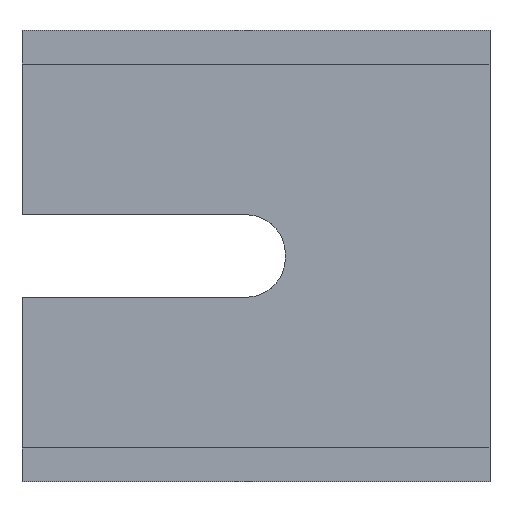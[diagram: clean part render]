
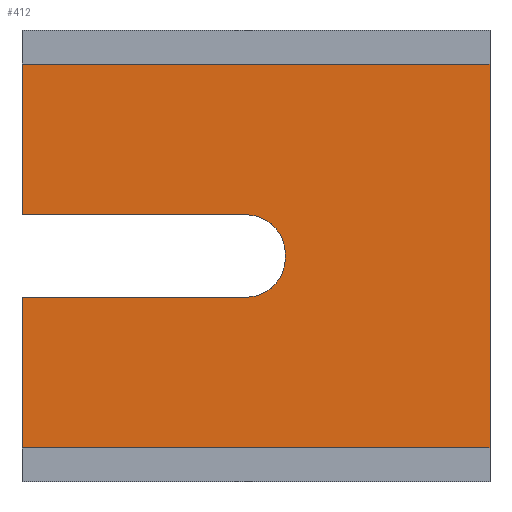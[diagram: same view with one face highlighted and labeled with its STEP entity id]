
A CAD part, front view. The second image highlights one B-rep face of the part: STEP entity #412.
In plain terms, the highlighted planar face has unit normal (0, -1, 0).
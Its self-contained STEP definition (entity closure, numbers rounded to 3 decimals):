
#28=CIRCLE('',#443,2.);
#30=CIRCLE('',#447,2.);
#52=FACE_OUTER_BOUND('',#76,.T.);
#76=EDGE_LOOP('',(#365,#366,#367,#368,#369,#370,#371,#372,#373,#374));
#91=LINE('',#595,#137);
#98=LINE('',#611,#144);
#106=LINE('',#627,#152);
#109=LINE('',#638,#155);
#115=LINE('',#665,#161);
#120=LINE('',#686,#166);
#121=LINE('',#688,#167);
#122=LINE('',#691,#168);
#137=VECTOR('',#480,10.);
#144=VECTOR('',#493,10.);
#152=VECTOR('',#509,10.);
#155=VECTOR('',#518,10.);
#161=VECTOR('',#534,10.);
#166=VECTOR('',#547,10.);
#167=VECTOR('',#550,10.);
#168=VECTOR('',#555,10.);
#181=VERTEX_POINT('',#592);
#182=VERTEX_POINT('',#594);
#187=VERTEX_POINT('',#608);
#188=VERTEX_POINT('',#610);
#196=VERTEX_POINT('',#635);
#197=VERTEX_POINT('',#637);
#200=VERTEX_POINT('',#655);
#201=VERTEX_POINT('',#657);
#203=VERTEX_POINT('',#663);
#204=VERTEX_POINT('',#667);
#221=EDGE_CURVE('',#181,#182,#91,.T.);
#229=EDGE_CURVE('',#188,#187,#98,.T.);
#238=EDGE_CURVE('',#188,#181,#106,.T.);
#243=EDGE_CURVE('',#196,#197,#109,.T.);
#248=EDGE_CURVE('',#200,#201,#28,.T.);
#252=EDGE_CURVE('',#200,#203,#115,.T.);
#253=EDGE_CURVE('',#204,#203,#30,.T.);
#259=EDGE_CURVE('',#204,#182,#120,.T.);
#260=EDGE_CURVE('',#196,#201,#121,.T.);
#261=EDGE_CURVE('',#197,#187,#122,.T.);
#365=ORIENTED_EDGE('',*,*,#259,.T.);
#366=ORIENTED_EDGE('',*,*,#221,.F.);
#367=ORIENTED_EDGE('',*,*,#238,.F.);
#368=ORIENTED_EDGE('',*,*,#229,.T.);
#369=ORIENTED_EDGE('',*,*,#261,.F.);
#370=ORIENTED_EDGE('',*,*,#243,.F.);
#371=ORIENTED_EDGE('',*,*,#260,.T.);
#372=ORIENTED_EDGE('',*,*,#248,.F.);
#373=ORIENTED_EDGE('',*,*,#252,.T.);
#374=ORIENTED_EDGE('',*,*,#253,.F.);
#391=PLANE('',#455);
#412=ADVANCED_FACE('',(#52),#391,.T.);
#443=AXIS2_PLACEMENT_3D('',#658,#526,#527);
#447=AXIS2_PLACEMENT_3D('',#668,#537,#538);
#455=AXIS2_PLACEMENT_3D('',#695,#560,#561);
#480=DIRECTION('',(0.,0.,1.));
#493=DIRECTION('',(0.,0.,1.));
#509=DIRECTION('',(-1.,0.,0.));
#518=DIRECTION('',(0.,0.,1.));
#526=DIRECTION('center_axis',(0.,-1.,0.));
#527=DIRECTION('ref_axis',(0.707,0.,0.707));
#534=DIRECTION('',(0.,0.,-1.));
#537=DIRECTION('center_axis',(0.,-1.,0.));
#538=DIRECTION('ref_axis',(0.707,0.,-0.707));
#547=DIRECTION('',(-1.,0.,0.));
#550=DIRECTION('',(1.,0.,0.));
#555=DIRECTION('',(1.,0.,0.));
#560=DIRECTION('center_axis',(0.,-1.,0.));
#561=DIRECTION('ref_axis',(1.,0.,0.));
#592=CARTESIAN_POINT('',(103.995,-15.75,-9.786));
#594=CARTESIAN_POINT('',(103.995,-15.75,-2.1));
#595=CARTESIAN_POINT('',(103.995,-15.75,0.));
#608=CARTESIAN_POINT('',(127.85,-15.75,9.786));
#610=CARTESIAN_POINT('',(127.85,-15.75,-9.786));
#611=CARTESIAN_POINT('',(127.85,-15.75,0.));
#627=CARTESIAN_POINT('',(127.85,-15.75,-9.786));
#635=CARTESIAN_POINT('',(103.995,-15.75,2.1));
#637=CARTESIAN_POINT('',(103.995,-15.75,9.786));
#638=CARTESIAN_POINT('',(103.995,-15.75,0.));
#655=CARTESIAN_POINT('',(117.419,-15.75,0.1));
#657=CARTESIAN_POINT('',(115.419,-15.75,2.1));
#658=CARTESIAN_POINT('Origin',(115.419,-15.75,0.1));
#663=CARTESIAN_POINT('',(117.419,-15.75,-0.1));
#665=CARTESIAN_POINT('',(117.419,-15.75,1.05));
#667=CARTESIAN_POINT('',(115.419,-15.75,-2.1));
#668=CARTESIAN_POINT('Origin',(115.419,-15.75,-0.1));
#686=CARTESIAN_POINT('',(109.707,-15.75,-2.1));
#688=CARTESIAN_POINT('',(109.707,-15.75,2.1));
#691=CARTESIAN_POINT('',(127.85,-15.75,9.786));
#695=CARTESIAN_POINT('Origin',(103.995,-15.75,0.));
